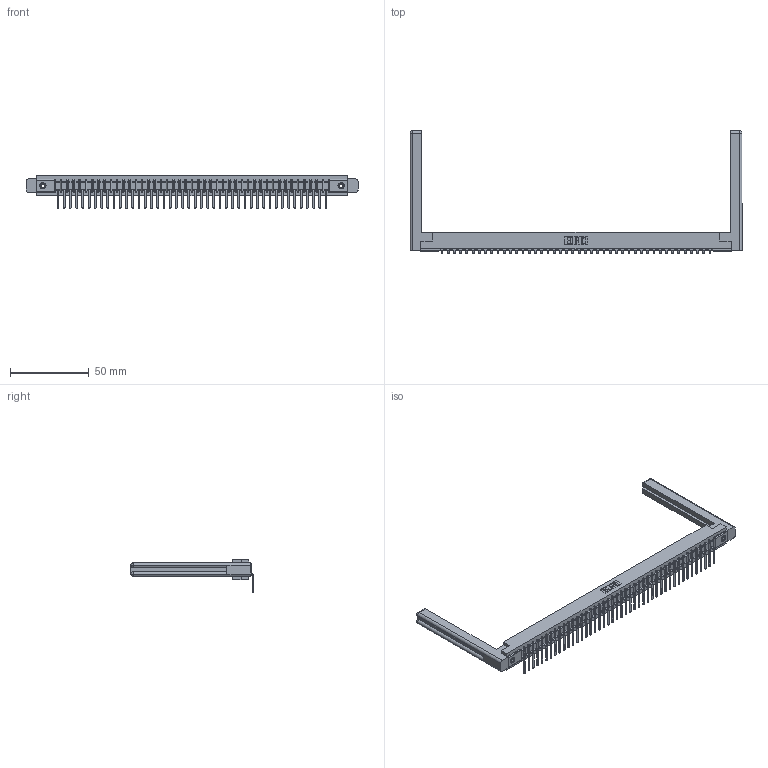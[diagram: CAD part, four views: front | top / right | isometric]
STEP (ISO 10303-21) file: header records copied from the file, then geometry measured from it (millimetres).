
FILE_DESCRIPTION (( 'STEP AP203' ), '1' );
FILE_NAME ('357-044-557-158.STEP', '2019-09-17T12:05:02', ( '' ), ( '' ), 'SwSTEP 2.0', 'SolidWorks 2016', '' );
FILE_SCHEMA (( 'CONFIG_CONTROL_DESIGN' ));
Length unit declared in the file: inch
Products named in the file (5): 357-044-557-158; 307-290-002_557; 307-220-058; 345-250-001_345-250-001-102; 307 Part_.156 Dia Mounting Holes
Assembly tree (49 placements, depth 2):
  357-044-557-158
    307 Part_.156 Dia Mounting Holes
    307-290-002_557  x44
    307-220-058  x2
    345-250-001_345-250-001-102  x2
Bounding box: 210.97 x 77.64 x 20.66 mm (x, y, z)
Volume: 29830.6 mm3; surface area: 34202.3 mm2
Topology: 49 solids, 49 shells, 3737 faces, 11413 edges, 7474 vertices
Faces by surface type: plane 2222, cylinder 1401, sphere 90, torus 12, cone 12
Entity records: 40961 total; most frequent: CARTESIAN_POINT 6919, ORIENTED_EDGE 6848, DIRECTION 6682, EDGE_CURVE 3424, VECTOR 2620, LINE 2620, VERTEX_POINT 2214, AXIS2_PLACEMENT_3D 2031
